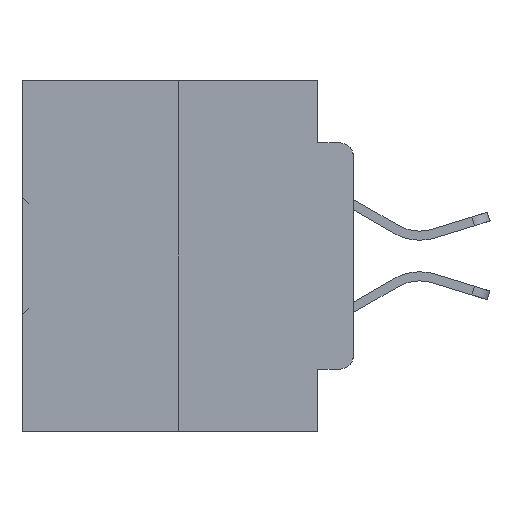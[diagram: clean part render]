
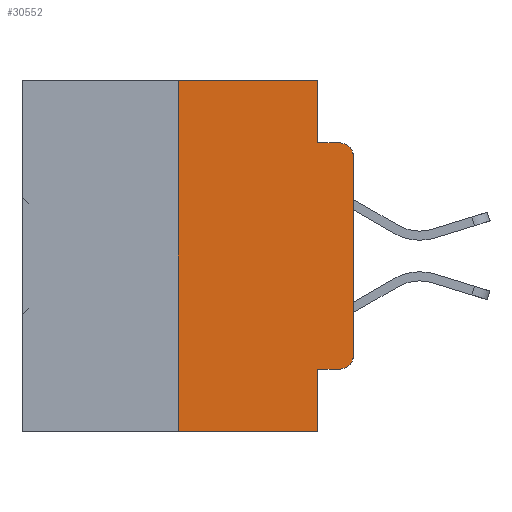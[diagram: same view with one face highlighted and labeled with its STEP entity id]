
A CAD part, left-side view. The second image highlights one B-rep face of the part: STEP entity #30552.
In plain terms, the highlighted planar face has unit normal (-1, 0, 0).
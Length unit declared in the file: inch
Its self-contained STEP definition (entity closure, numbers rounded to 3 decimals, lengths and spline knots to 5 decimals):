
#91 = AXIS2_PLACEMENT_3D ( 'NONE', #37744, #13526, #4730 ) ;
#329 = CARTESIAN_POINT ( 'NONE',  ( 0., 0.051, 0. ) ) ;
#823 = LINE ( 'NONE', #329, #38658 ) ;
#859 = VERTEX_POINT ( 'NONE', #6821 ) ;
#1724 = ORIENTED_EDGE ( 'NONE', *, *, #16670, .F. ) ;
#3125 = VERTEX_POINT ( 'NONE', #11887 ) ;
#3276 = ORIENTED_EDGE ( 'NONE', *, *, #4875, .F. ) ;
#4058 = LINE ( 'NONE', #8147, #28850 ) ;
#4730 = DIRECTION ( 'NONE',  ( 0., 0., -1. ) ) ;
#4875 = EDGE_CURVE ( 'NONE', #859, #37890, #9300, .T. ) ;
#5431 = DIRECTION ( 'NONE',  ( 0., 0., -1. ) ) ;
#5656 = CARTESIAN_POINT ( 'NONE',  ( 0., 0.051, -0.5 ) ) ;
#5762 = AXIS2_PLACEMENT_3D ( 'NONE', #16956, #29044, #8128 ) ;
#6502 = ORIENTED_EDGE ( 'NONE', *, *, #31227, .F. ) ;
#6742 = EDGE_CURVE ( 'NONE', #10279, #18016, #29212, .T. ) ;
#6821 = CARTESIAN_POINT ( 'NONE',  ( 0., 0.25, 0. ) ) ;
#7286 = VERTEX_POINT ( 'NONE', #7607 ) ;
#7607 = CARTESIAN_POINT ( 'NONE',  ( 0., 0.051, -0.4115 ) ) ;
#7795 = DIRECTION ( 'NONE',  ( -1., 0., 0. ) ) ;
#8030 = DIRECTION ( 'NONE',  ( 0., -1., 0. ) ) ;
#8128 = DIRECTION ( 'NONE',  ( 0., 0., -1. ) ) ;
#8147 = CARTESIAN_POINT ( 'NONE',  ( 0., 0.473, -0.5 ) ) ;
#8422 = CARTESIAN_POINT ( 'NONE',  ( 0., 0.051, -0.4115 ) ) ;
#8641 = VERTEX_POINT ( 'NONE', #19937 ) ;
#9300 = LINE ( 'NONE', #34913, #21956 ) ;
#9809 = AXIS2_PLACEMENT_3D ( 'NONE', #37692, #7795, #10844 ) ;
#10279 = VERTEX_POINT ( 'NONE', #12501 ) ;
#10844 = DIRECTION ( 'NONE',  ( 0., 0., -1. ) ) ;
#11887 = CARTESIAN_POINT ( 'NONE',  ( 0., 0.02, -0.0885 ) ) ;
#12501 = CARTESIAN_POINT ( 'NONE',  ( 0., 0.02, -0.4115 ) ) ;
#12908 = VERTEX_POINT ( 'NONE', #28585 ) ;
#13346 = CARTESIAN_POINT ( 'NONE',  ( 0., 0., -0.3915 ) ) ;
#13526 = DIRECTION ( 'NONE',  ( 1., 0., 0. ) ) ;
#13666 = ORIENTED_EDGE ( 'NONE', *, *, #29725, .F. ) ;
#13838 = VERTEX_POINT ( 'NONE', #5656 ) ;
#15368 = ORIENTED_EDGE ( 'NONE', *, *, #33765, .T. ) ;
#15398 = DIRECTION ( 'NONE',  ( 0., 0., -1. ) ) ;
#15571 = LINE ( 'NONE', #23394, #32836 ) ;
#16384 = VERTEX_POINT ( 'NONE', #35974 ) ;
#16508 = ORIENTED_EDGE ( 'NONE', *, *, #6742, .T. ) ;
#16670 = EDGE_CURVE ( 'NONE', #16384, #859, #34821, .T. ) ;
#16956 = CARTESIAN_POINT ( 'NONE',  ( 0., 0.02, -0.1085 ) ) ;
#17243 = ORIENTED_EDGE ( 'NONE', *, *, #30079, .T. ) ;
#17580 = ORIENTED_EDGE ( 'NONE', *, *, #34497, .T. ) ;
#17586 = DIRECTION ( 'NONE',  ( 0., 0., 1. ) ) ;
#17622 = VECTOR ( 'NONE', #33496, 39.37008 ) ;
#18016 = VERTEX_POINT ( 'NONE', #13346 ) ;
#19528 = CARTESIAN_POINT ( 'NONE',  ( 0., 0.051, 0. ) ) ;
#19933 = VECTOR ( 'NONE', #20003, 39.37008 ) ;
#19937 = CARTESIAN_POINT ( 'NONE',  ( 0., 0.051, -0.0885 ) ) ;
#20003 = DIRECTION ( 'NONE',  ( 0., -1., 0. ) ) ;
#21956 = VECTOR ( 'NONE', #29063, 39.37008 ) ;
#23283 = FACE_OUTER_BOUND ( 'NONE', #29477, .T. ) ;
#23394 = CARTESIAN_POINT ( 'NONE',  ( 0., 0.051, 0. ) ) ;
#24856 = ORIENTED_EDGE ( 'NONE', *, *, #37946, .T. ) ;
#25651 = CIRCLE ( 'NONE', #5762, 0.02 ) ;
#25994 = LINE ( 'NONE', #31978, #19933 ) ;
#26697 = CARTESIAN_POINT ( 'NONE',  ( 0., 0., 0. ) ) ;
#27391 = CARTESIAN_POINT ( 'NONE',  ( 0., 0.25, 0. ) ) ;
#27660 = LINE ( 'NONE', #8422, #29551 ) ;
#28585 = CARTESIAN_POINT ( 'NONE',  ( 0., 0., -0.1085 ) ) ;
#28850 = VECTOR ( 'NONE', #8030, 39.37008 ) ;
#29044 = DIRECTION ( 'NONE',  ( -1., 0., 0. ) ) ;
#29063 = DIRECTION ( 'NONE',  ( 0., -1., 0. ) ) ;
#29212 = CIRCLE ( 'NONE', #9809, 0.02 ) ;
#29477 = EDGE_LOOP ( 'NONE', ( #17580, #24856, #6502, #13666, #3276, #1724, #17243, #34578, #15368, #16508 ) ) ;
#29551 = VECTOR ( 'NONE', #38171, 39.37008 ) ;
#29725 = EDGE_CURVE ( 'NONE', #37890, #8641, #823, .T. ) ;
#30079 = EDGE_CURVE ( 'NONE', #16384, #13838, #4058, .T. ) ;
#30552 = ADVANCED_FACE ( 'NONE', ( #23283 ), #31619, .F. ) ;
#31025 = VECTOR ( 'NONE', #17586, 39.37008 ) ;
#31209 = LINE ( 'NONE', #26697, #31025 ) ;
#31227 = EDGE_CURVE ( 'NONE', #8641, #3125, #25994, .T. ) ;
#31619 = PLANE ( 'NONE',  #91 ) ;
#31978 = CARTESIAN_POINT ( 'NONE',  ( 0., 0.051, -0.0885 ) ) ;
#32836 = VECTOR ( 'NONE', #5431, 39.37008 ) ;
#33496 = DIRECTION ( 'NONE',  ( 0., 0., 1. ) ) ;
#33765 = EDGE_CURVE ( 'NONE', #7286, #10279, #27660, .T. ) ;
#34497 = EDGE_CURVE ( 'NONE', #18016, #12908, #31209, .T. ) ;
#34578 = ORIENTED_EDGE ( 'NONE', *, *, #35654, .F. ) ;
#34821 = LINE ( 'NONE', #27391, #17622 ) ;
#34913 = CARTESIAN_POINT ( 'NONE',  ( 0., 0.473, 0. ) ) ;
#35654 = EDGE_CURVE ( 'NONE', #7286, #13838, #15571, .T. ) ;
#35974 = CARTESIAN_POINT ( 'NONE',  ( 0., 0.25, -0.5 ) ) ;
#37692 = CARTESIAN_POINT ( 'NONE',  ( 0., 0.02, -0.3915 ) ) ;
#37744 = CARTESIAN_POINT ( 'NONE',  ( 0., 0.473, 0. ) ) ;
#37890 = VERTEX_POINT ( 'NONE', #19528 ) ;
#37946 = EDGE_CURVE ( 'NONE', #12908, #3125, #25651, .T. ) ;
#38171 = DIRECTION ( 'NONE',  ( 0., -1., 0. ) ) ;
#38658 = VECTOR ( 'NONE', #15398, 39.37008 ) ;
